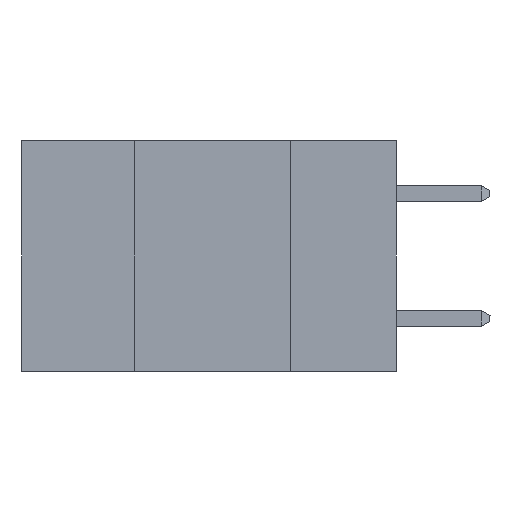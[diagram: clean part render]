
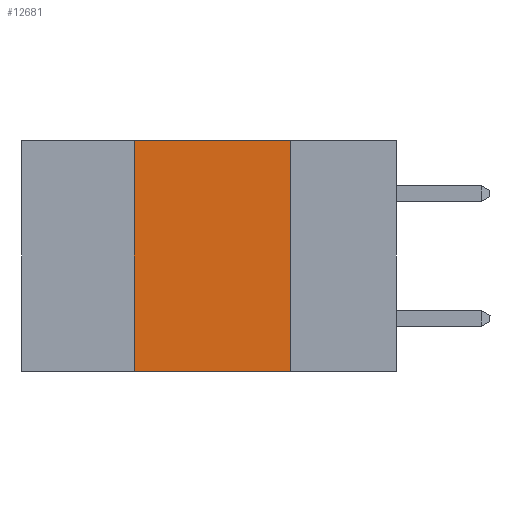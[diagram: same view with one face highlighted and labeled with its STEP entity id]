
A CAD part, left-side view. The second image highlights one B-rep face of the part: STEP entity #12681.
In plain terms, the highlighted planar face has unit normal (-1, 0, 0).
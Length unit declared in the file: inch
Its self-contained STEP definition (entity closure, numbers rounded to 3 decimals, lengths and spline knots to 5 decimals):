
#9 = FACE_OUTER_BOUND ( 'NONE', #17588, .T. ) ;
#75 = LINE ( 'NONE', #2460, #20246 ) ;
#432 = DIRECTION ( 'NONE',  ( 1., 0., 0. ) ) ;
#802 = EDGE_CURVE ( 'NONE', #25114, #16995, #13862, .T. ) ;
#1838 = CARTESIAN_POINT ( 'NONE',  ( 0., 0.6, 0. ) ) ;
#2230 = ORIENTED_EDGE ( 'NONE', *, *, #16847, .F. ) ;
#2460 = CARTESIAN_POINT ( 'NONE',  ( 0., 0.17, -0.37 ) ) ;
#3965 = EDGE_CURVE ( 'NONE', #25114, #10266, #23673, .T. ) ;
#4196 = ORIENTED_EDGE ( 'NONE', *, *, #3965, .F. ) ;
#4801 = CARTESIAN_POINT ( 'NONE',  ( 0., 0.17, 0. ) ) ;
#8090 = CARTESIAN_POINT ( 'NONE',  ( 0., 0.42, -0.37 ) ) ;
#8308 = PLANE ( 'NONE',  #15293 ) ;
#8442 = ORIENTED_EDGE ( 'NONE', *, *, #11381, .F. ) ;
#9166 = ORIENTED_EDGE ( 'NONE', *, *, #802, .T. ) ;
#10266 = VERTEX_POINT ( 'NONE', #23489 ) ;
#11381 = EDGE_CURVE ( 'NONE', #14485, #16995, #75, .T. ) ;
#11514 = VECTOR ( 'NONE', #11656, 39.37008 ) ;
#11656 = DIRECTION ( 'NONE',  ( 0., -1., 0. ) ) ;
#12189 = CARTESIAN_POINT ( 'NONE',  ( 0., 0.6, 0. ) ) ;
#12328 = DIRECTION ( 'NONE',  ( 0., 0., -1. ) ) ;
#12469 = CARTESIAN_POINT ( 'NONE',  ( 0., 0.17, -0.37 ) ) ;
#12681 = ADVANCED_FACE ( 'NONE', ( #9 ), #8308, .F. ) ;
#13417 = VECTOR ( 'NONE', #14998, 39.37008 ) ;
#13862 = LINE ( 'NONE', #22064, #18422 ) ;
#14132 = DIRECTION ( 'NONE',  ( 0., 0., -1. ) ) ;
#14485 = VERTEX_POINT ( 'NONE', #4801 ) ;
#14998 = DIRECTION ( 'NONE',  ( 0., 0., 1. ) ) ;
#15293 = AXIS2_PLACEMENT_3D ( 'NONE', #12189, #432, #14132 ) ;
#16847 = EDGE_CURVE ( 'NONE', #10266, #14485, #17280, .T. ) ;
#16995 = VERTEX_POINT ( 'NONE', #12469 ) ;
#17080 = CARTESIAN_POINT ( 'NONE',  ( 0., 0.42, -0.37 ) ) ;
#17280 = LINE ( 'NONE', #1838, #11514 ) ;
#17588 = EDGE_LOOP ( 'NONE', ( #8442, #2230, #4196, #9166 ) ) ;
#18422 = VECTOR ( 'NONE', #22148, 39.37008 ) ;
#20246 = VECTOR ( 'NONE', #12328, 39.37008 ) ;
#22064 = CARTESIAN_POINT ( 'NONE',  ( 0., 0.6, -0.37 ) ) ;
#22148 = DIRECTION ( 'NONE',  ( 0., -1., 0. ) ) ;
#23489 = CARTESIAN_POINT ( 'NONE',  ( 0., 0.42, 0. ) ) ;
#23673 = LINE ( 'NONE', #17080, #13417 ) ;
#25114 = VERTEX_POINT ( 'NONE', #8090 ) ;
